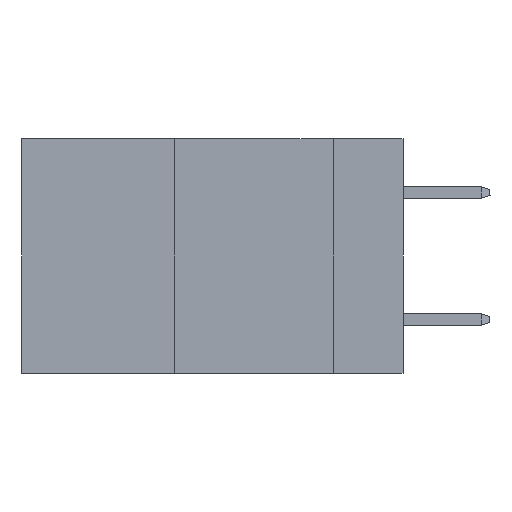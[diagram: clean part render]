
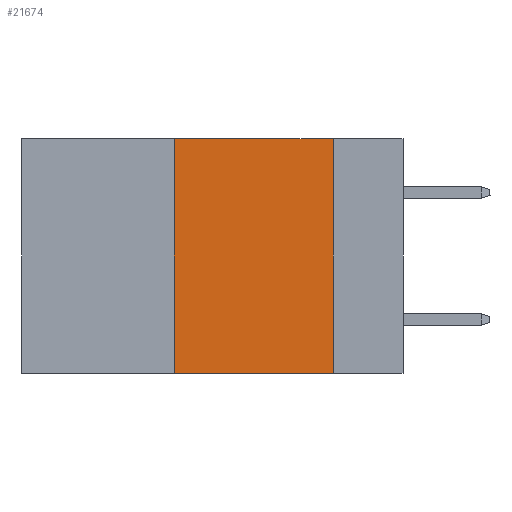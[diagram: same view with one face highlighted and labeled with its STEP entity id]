
A CAD part, left-side view. The second image highlights one B-rep face of the part: STEP entity #21674.
In plain terms, the highlighted planar face has unit normal (-1, 0, 0).
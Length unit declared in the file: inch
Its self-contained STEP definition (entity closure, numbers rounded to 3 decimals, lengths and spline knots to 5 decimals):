
#118 = DIRECTION ( 'NONE',  ( 0., -1., 0. ) ) ;
#1804 = PLANE ( 'NONE',  #43913 ) ;
#2298 = DIRECTION ( 'NONE',  ( 0., -1., 0. ) ) ;
#3825 = CARTESIAN_POINT ( 'NONE',  ( 0., 0.6, 0. ) ) ;
#4833 = CARTESIAN_POINT ( 'NONE',  ( 0., 0.11, 0. ) ) ;
#5106 = EDGE_CURVE ( 'NONE', #41494, #14520, #15775, .T. ) ;
#5726 = FACE_OUTER_BOUND ( 'NONE', #21957, .T. ) ;
#5773 = CARTESIAN_POINT ( 'NONE',  ( 0., 0.6, -0.37 ) ) ;
#7331 = CARTESIAN_POINT ( 'NONE',  ( 0., 0.36, 0. ) ) ;
#7662 = VERTEX_POINT ( 'NONE', #11221 ) ;
#11221 = CARTESIAN_POINT ( 'NONE',  ( 0., 0.36, -0.37 ) ) ;
#11909 = VECTOR ( 'NONE', #44277, 39.37008 ) ;
#14520 = VERTEX_POINT ( 'NONE', #35798 ) ;
#15775 = LINE ( 'NONE', #4833, #11909 ) ;
#17134 = LINE ( 'NONE', #7331, #20402 ) ;
#17191 = ORIENTED_EDGE ( 'NONE', *, *, #29059, .T. ) ;
#17863 = ORIENTED_EDGE ( 'NONE', *, *, #45044, .F. ) ;
#20402 = VECTOR ( 'NONE', #45862, 39.37008 ) ;
#20427 = DIRECTION ( 'NONE',  ( 0., 0., -1. ) ) ;
#21674 = ADVANCED_FACE ( 'NONE', ( #5726 ), #1804, .F. ) ;
#21957 = EDGE_LOOP ( 'NONE', ( #23857, #17863, #44753, #17191 ) ) ;
#22257 = VECTOR ( 'NONE', #118, 39.37008 ) ;
#23450 = VECTOR ( 'NONE', #2298, 39.37008 ) ;
#23857 = ORIENTED_EDGE ( 'NONE', *, *, #5106, .F. ) ;
#24430 = EDGE_CURVE ( 'NONE', #7662, #44000, #17134, .T. ) ;
#26339 = CARTESIAN_POINT ( 'NONE',  ( 0., 0.11, 0. ) ) ;
#27205 = DIRECTION ( 'NONE',  ( 1., 0., 0. ) ) ;
#29059 = EDGE_CURVE ( 'NONE', #7662, #14520, #44991, .T. ) ;
#34030 = CARTESIAN_POINT ( 'NONE',  ( 0., 0.6, 0. ) ) ;
#35798 = CARTESIAN_POINT ( 'NONE',  ( 0., 0.11, -0.37 ) ) ;
#36250 = CARTESIAN_POINT ( 'NONE',  ( 0., 0.36, 0. ) ) ;
#41494 = VERTEX_POINT ( 'NONE', #26339 ) ;
#43913 = AXIS2_PLACEMENT_3D ( 'NONE', #34030, #27205, #20427 ) ;
#44000 = VERTEX_POINT ( 'NONE', #36250 ) ;
#44277 = DIRECTION ( 'NONE',  ( 0., 0., -1. ) ) ;
#44753 = ORIENTED_EDGE ( 'NONE', *, *, #24430, .F. ) ;
#44991 = LINE ( 'NONE', #5773, #23450 ) ;
#45044 = EDGE_CURVE ( 'NONE', #44000, #41494, #45843, .T. ) ;
#45843 = LINE ( 'NONE', #3825, #22257 ) ;
#45862 = DIRECTION ( 'NONE',  ( 0., 0., 1. ) ) ;
